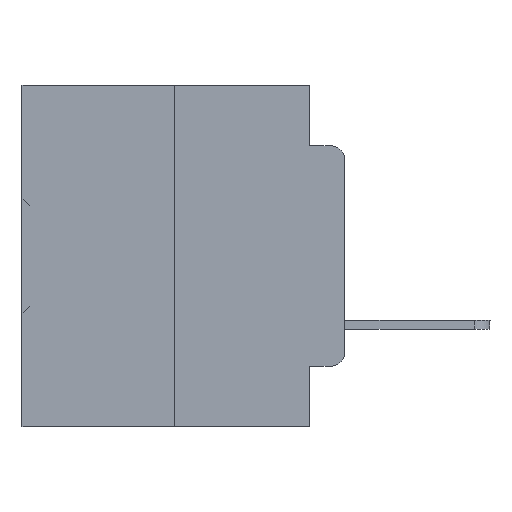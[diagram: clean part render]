
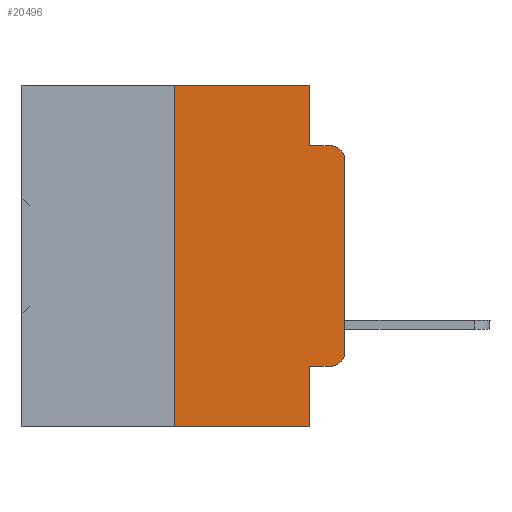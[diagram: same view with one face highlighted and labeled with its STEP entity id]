
A CAD part, left-side view. The second image highlights one B-rep face of the part: STEP entity #20496.
In plain terms, the highlighted planar face has unit normal (-1, 0, 0).
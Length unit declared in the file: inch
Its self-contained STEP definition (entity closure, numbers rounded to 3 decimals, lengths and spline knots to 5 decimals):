
#207 = ORIENTED_EDGE ( 'NONE', *, *, #21272, .T. ) ;
#925 = CARTESIAN_POINT ( 'NONE',  ( 0., 0.051, -0.5 ) ) ;
#2354 = CARTESIAN_POINT ( 'NONE',  ( 0., 0.473, 0. ) ) ;
#3412 = EDGE_CURVE ( 'NONE', #12018, #35586, #34359, .T. ) ;
#3583 = VERTEX_POINT ( 'NONE', #21659 ) ;
#4434 = CARTESIAN_POINT ( 'NONE',  ( 0., 0.051, 0. ) ) ;
#5020 = CARTESIAN_POINT ( 'NONE',  ( 0., 0.25, -0.5 ) ) ;
#6090 = CARTESIAN_POINT ( 'NONE',  ( 0., 0.02, -0.4115 ) ) ;
#6104 = EDGE_CURVE ( 'NONE', #12018, #29381, #36017, .T. ) ;
#6708 = VERTEX_POINT ( 'NONE', #5020 ) ;
#6914 = EDGE_CURVE ( 'NONE', #10288, #35546, #15942, .T. ) ;
#7625 = CARTESIAN_POINT ( 'NONE',  ( 0., 0., 0. ) ) ;
#8184 = CARTESIAN_POINT ( 'NONE',  ( 0., 0.051, -0.4115 ) ) ;
#8397 = ORIENTED_EDGE ( 'NONE', *, *, #31488, .F. ) ;
#8919 = CARTESIAN_POINT ( 'NONE',  ( 0., 0.051, -0.0885 ) ) ;
#8989 = PLANE ( 'NONE',  #24699 ) ;
#9225 = CARTESIAN_POINT ( 'NONE',  ( 0., 0., -0.1085 ) ) ;
#10288 = VERTEX_POINT ( 'NONE', #22796 ) ;
#10965 = DIRECTION ( 'NONE',  ( 0., 0., -1. ) ) ;
#11169 = CIRCLE ( 'NONE', #32564, 0.02 ) ;
#11307 = CARTESIAN_POINT ( 'NONE',  ( 0., 0.051, -0.0885 ) ) ;
#11435 = LINE ( 'NONE', #23721, #23580 ) ;
#12018 = VERTEX_POINT ( 'NONE', #25561 ) ;
#12273 = DIRECTION ( 'NONE',  ( 0., -1., 0. ) ) ;
#12555 = DIRECTION ( 'NONE',  ( 0., 0., -1. ) ) ;
#14114 = ORIENTED_EDGE ( 'NONE', *, *, #14335, .T. ) ;
#14335 = EDGE_CURVE ( 'NONE', #17388, #31719, #23562, .T. ) ;
#14351 = DIRECTION ( 'NONE',  ( 1., 0., 0. ) ) ;
#14543 = AXIS2_PLACEMENT_3D ( 'NONE', #27347, #24358, #35762 ) ;
#15303 = VERTEX_POINT ( 'NONE', #11307 ) ;
#15534 = CARTESIAN_POINT ( 'NONE',  ( 0., 0.051, 0. ) ) ;
#15942 = LINE ( 'NONE', #26411, #20159 ) ;
#17273 = CARTESIAN_POINT ( 'NONE',  ( 0., 0.25, 0. ) ) ;
#17296 = DIRECTION ( 'NONE',  ( 0., -1., 0. ) ) ;
#17388 = VERTEX_POINT ( 'NONE', #9225 ) ;
#18402 = LINE ( 'NONE', #17273, #31965 ) ;
#18509 = EDGE_LOOP ( 'NONE', ( #22280, #14114, #8397, #35261, #22882, #33726, #207, #34420, #33600, #31983 ) ) ;
#20159 = VECTOR ( 'NONE', #12273, 39.37008 ) ;
#20496 = ADVANCED_FACE ( 'NONE', ( #25511 ), #8989, .F. ) ;
#21272 = EDGE_CURVE ( 'NONE', #6708, #35586, #11435, .T. ) ;
#21659 = CARTESIAN_POINT ( 'NONE',  ( 0., 0., -0.3915 ) ) ;
#21732 = EDGE_CURVE ( 'NONE', #6708, #10288, #18402, .T. ) ;
#22280 = ORIENTED_EDGE ( 'NONE', *, *, #27432, .T. ) ;
#22796 = CARTESIAN_POINT ( 'NONE',  ( 0., 0.25, 0. ) ) ;
#22882 = ORIENTED_EDGE ( 'NONE', *, *, #6914, .F. ) ;
#23562 = CIRCLE ( 'NONE', #14543, 0.02 ) ;
#23580 = VECTOR ( 'NONE', #35772, 39.37008 ) ;
#23721 = CARTESIAN_POINT ( 'NONE',  ( 0., 0.473, -0.5 ) ) ;
#23930 = LINE ( 'NONE', #8919, #28601 ) ;
#24358 = DIRECTION ( 'NONE',  ( -1., 0., 0. ) ) ;
#24564 = DIRECTION ( 'NONE',  ( -1., 0., 0. ) ) ;
#24699 = AXIS2_PLACEMENT_3D ( 'NONE', #2354, #14351, #10965 ) ;
#24948 = DIRECTION ( 'NONE',  ( 0., 0., -1. ) ) ;
#25511 = FACE_OUTER_BOUND ( 'NONE', #18509, .T. ) ;
#25561 = CARTESIAN_POINT ( 'NONE',  ( 0., 0.051, -0.4115 ) ) ;
#26196 = EDGE_CURVE ( 'NONE', #35546, #15303, #26231, .T. ) ;
#26231 = LINE ( 'NONE', #4434, #27604 ) ;
#26411 = CARTESIAN_POINT ( 'NONE',  ( 0., 0.473, 0. ) ) ;
#27042 = VECTOR ( 'NONE', #28604, 39.37008 ) ;
#27347 = CARTESIAN_POINT ( 'NONE',  ( 0., 0.02, -0.1085 ) ) ;
#27432 = EDGE_CURVE ( 'NONE', #3583, #17388, #27970, .T. ) ;
#27604 = VECTOR ( 'NONE', #28052, 39.37008 ) ;
#27970 = LINE ( 'NONE', #7625, #27042 ) ;
#28052 = DIRECTION ( 'NONE',  ( 0., 0., -1. ) ) ;
#28144 = VECTOR ( 'NONE', #17296, 39.37008 ) ;
#28601 = VECTOR ( 'NONE', #30044, 39.37008 ) ;
#28604 = DIRECTION ( 'NONE',  ( 0., 0., 1. ) ) ;
#29381 = VERTEX_POINT ( 'NONE', #6090 ) ;
#30044 = DIRECTION ( 'NONE',  ( 0., -1., 0. ) ) ;
#31488 = EDGE_CURVE ( 'NONE', #15303, #31719, #23930, .T. ) ;
#31719 = VERTEX_POINT ( 'NONE', #37807 ) ;
#31965 = VECTOR ( 'NONE', #32024, 39.37008 ) ;
#31983 = ORIENTED_EDGE ( 'NONE', *, *, #36836, .T. ) ;
#32024 = DIRECTION ( 'NONE',  ( 0., 0., 1. ) ) ;
#32564 = AXIS2_PLACEMENT_3D ( 'NONE', #36618, #24564, #24948 ) ;
#33011 = CARTESIAN_POINT ( 'NONE',  ( 0., 0.051, 0. ) ) ;
#33600 = ORIENTED_EDGE ( 'NONE', *, *, #6104, .T. ) ;
#33726 = ORIENTED_EDGE ( 'NONE', *, *, #21732, .F. ) ;
#33917 = VECTOR ( 'NONE', #12555, 39.37008 ) ;
#34359 = LINE ( 'NONE', #15534, #33917 ) ;
#34420 = ORIENTED_EDGE ( 'NONE', *, *, #3412, .F. ) ;
#35261 = ORIENTED_EDGE ( 'NONE', *, *, #26196, .F. ) ;
#35546 = VERTEX_POINT ( 'NONE', #33011 ) ;
#35586 = VERTEX_POINT ( 'NONE', #925 ) ;
#35762 = DIRECTION ( 'NONE',  ( 0., 0., -1. ) ) ;
#35772 = DIRECTION ( 'NONE',  ( 0., -1., 0. ) ) ;
#36017 = LINE ( 'NONE', #8184, #28144 ) ;
#36618 = CARTESIAN_POINT ( 'NONE',  ( 0., 0.02, -0.3915 ) ) ;
#36836 = EDGE_CURVE ( 'NONE', #29381, #3583, #11169, .T. ) ;
#37807 = CARTESIAN_POINT ( 'NONE',  ( 0., 0.02, -0.0885 ) ) ;
